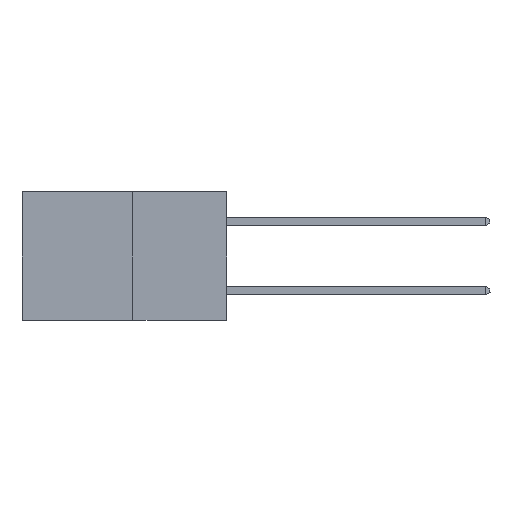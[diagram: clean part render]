
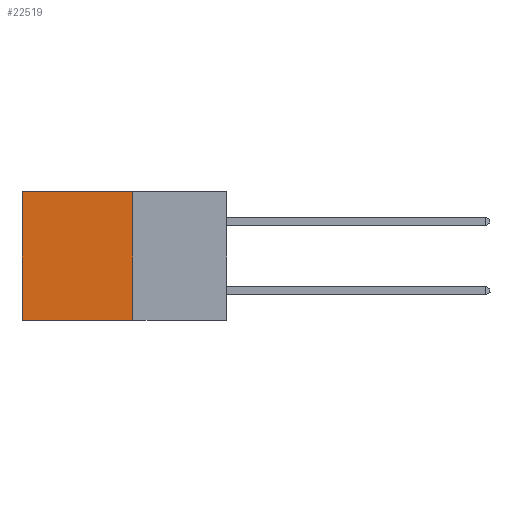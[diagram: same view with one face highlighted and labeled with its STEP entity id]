
A CAD part, left-side view. The second image highlights one B-rep face of the part: STEP entity #22519.
In plain terms, the highlighted planar face has unit normal (-1, 0, 0).
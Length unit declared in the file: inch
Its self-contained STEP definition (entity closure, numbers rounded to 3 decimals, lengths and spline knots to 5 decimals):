
#34 = ORIENTED_EDGE ( 'NONE', *, *, #3299, .T. ) ;
#521 = PLANE ( 'NONE',  #15918 ) ;
#1959 = LINE ( 'NONE', #22591, #12245 ) ;
#2004 = CARTESIAN_POINT ( 'NONE',  ( 0.277, 0.27, 0. ) ) ;
#2495 = DIRECTION ( 'NONE',  ( 1., 0., 0. ) ) ;
#3129 = CARTESIAN_POINT ( 'NONE',  ( 0.277, 0.59, -0.37 ) ) ;
#3299 = EDGE_CURVE ( 'NONE', #16215, #23440, #12345, .T. ) ;
#3798 = ORIENTED_EDGE ( 'NONE', *, *, #22133, .T. ) ;
#4106 = ORIENTED_EDGE ( 'NONE', *, *, #17244, .F. ) ;
#5188 = LINE ( 'NONE', #18632, #24338 ) ;
#6883 = CARTESIAN_POINT ( 'NONE',  ( 0.277, 0.59, -0.37 ) ) ;
#8127 = DIRECTION ( 'NONE',  ( 0., 0., -1. ) ) ;
#8360 = ORIENTED_EDGE ( 'NONE', *, *, #12308, .F. ) ;
#10516 = CARTESIAN_POINT ( 'NONE',  ( 0.277, 0.59, 0. ) ) ;
#11808 = VERTEX_POINT ( 'NONE', #17507 ) ;
#12245 = VECTOR ( 'NONE', #15023, 39.37008 ) ;
#12308 = EDGE_CURVE ( 'NONE', #11808, #23440, #1959, .T. ) ;
#12345 = LINE ( 'NONE', #3129, #21916 ) ;
#13643 = VERTEX_POINT ( 'NONE', #2004 ) ;
#14066 = CARTESIAN_POINT ( 'NONE',  ( 0.277, 0.27, -0.37 ) ) ;
#15023 = DIRECTION ( 'NONE',  ( 0., 1., 0. ) ) ;
#15136 = FACE_OUTER_BOUND ( 'NONE', #24017, .T. ) ;
#15918 = AXIS2_PLACEMENT_3D ( 'NONE', #14066, #2495, #16010 ) ;
#16010 = DIRECTION ( 'NONE',  ( 0., 0., -1. ) ) ;
#16215 = VERTEX_POINT ( 'NONE', #10516 ) ;
#16793 = DIRECTION ( 'NONE',  ( 0., 1., 0. ) ) ;
#17244 = EDGE_CURVE ( 'NONE', #13643, #11808, #18658, .T. ) ;
#17507 = CARTESIAN_POINT ( 'NONE',  ( 0.277, 0.27, -0.37 ) ) ;
#18068 = VECTOR ( 'NONE', #21324, 39.37008 ) ;
#18632 = CARTESIAN_POINT ( 'NONE',  ( 0.277, 0.27, 0. ) ) ;
#18658 = LINE ( 'NONE', #19439, #18068 ) ;
#19439 = CARTESIAN_POINT ( 'NONE',  ( 0.277, 0.27, -0.37 ) ) ;
#21324 = DIRECTION ( 'NONE',  ( 0., 0., -1. ) ) ;
#21916 = VECTOR ( 'NONE', #8127, 39.37008 ) ;
#22133 = EDGE_CURVE ( 'NONE', #13643, #16215, #5188, .T. ) ;
#22519 = ADVANCED_FACE ( 'NONE', ( #15136 ), #521, .F. ) ;
#22591 = CARTESIAN_POINT ( 'NONE',  ( 0.277, 0.27, -0.37 ) ) ;
#23440 = VERTEX_POINT ( 'NONE', #6883 ) ;
#24017 = EDGE_LOOP ( 'NONE', ( #34, #8360, #4106, #3798 ) ) ;
#24338 = VECTOR ( 'NONE', #16793, 39.37008 ) ;
